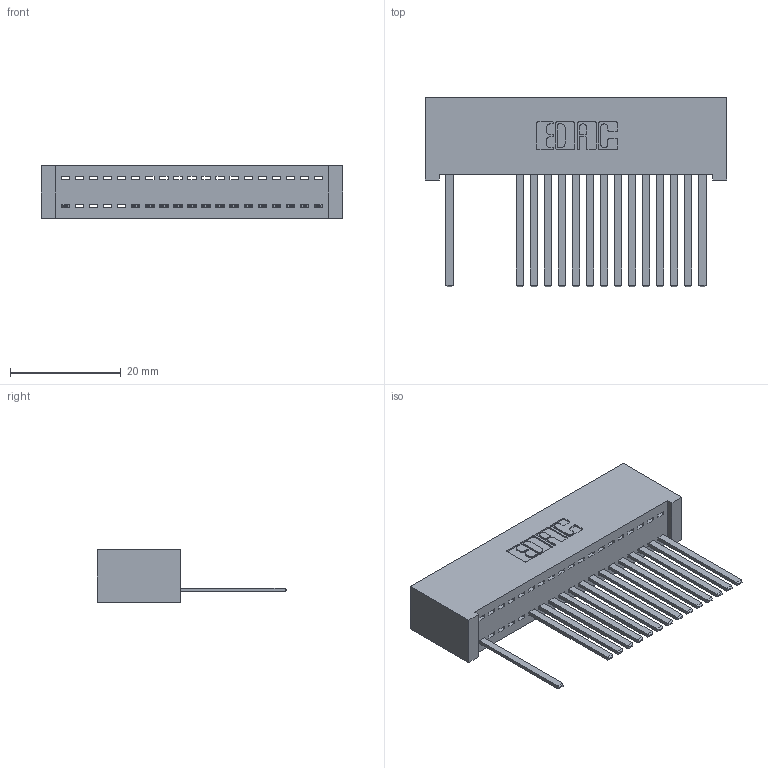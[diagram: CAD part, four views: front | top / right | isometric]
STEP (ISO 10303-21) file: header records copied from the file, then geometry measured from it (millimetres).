
FILE_DESCRIPTION (( 'STEP AP203' ), '1' );
FILE_NAME ('392-019-544-101.STEP', '2018-08-15T05:35:57', ( '' ), ( '' ), 'SwSTEP 2.0', 'SolidWorks 2016', '' );
FILE_SCHEMA (( 'CONFIG_CONTROL_DESIGN' ));
Length unit declared in the file: inch
Products named in the file (3): 392-019-544-101; 342 Part_Lugless; 345-292-001_345-293-144
Assembly tree (16 placements, depth 2):
  392-019-544-101
    342 Part_Lugless
    345-292-001_345-293-144  x15
Bounding box: 54.51 x 34.3 x 9.4 mm (x, y, z)
Volume: 5231.5 mm3; surface area: 7833.5 mm2
Topology: 16 solids, 16 shells, 930 faces, 2813 edges, 1854 vertices
Faces by surface type: plane 680, cylinder 250
Entity records: 13869 total; most frequent: CARTESIAN_POINT 2419, ORIENTED_EDGE 2378, DIRECTION 2071, EDGE_CURVE 1189, LINE 1073, VECTOR 1073, VERTEX_POINT 790, AXIS2_PLACEMENT_3D 499
